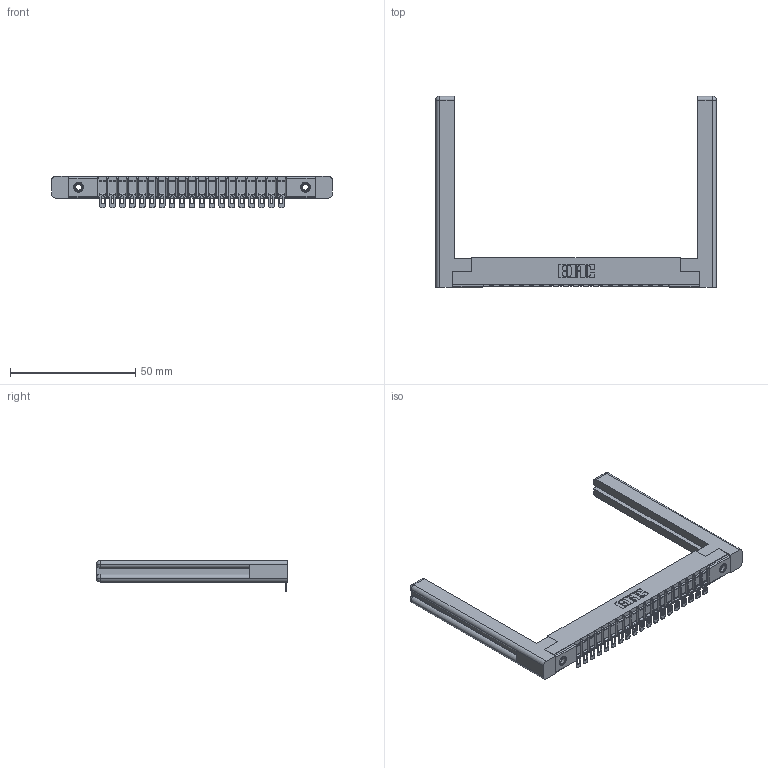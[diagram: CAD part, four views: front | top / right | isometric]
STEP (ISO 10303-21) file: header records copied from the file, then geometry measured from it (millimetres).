
FILE_DESCRIPTION (( 'STEP AP203' ), '1' );
FILE_NAME ('307-019-554-158.STEP', '2019-09-04T22:49:40', ( '' ), ( '' ), 'SwSTEP 2.0', 'SolidWorks 2016', '' );
FILE_SCHEMA (( 'CONFIG_CONTROL_DESIGN' ));
Length unit declared in the file: inch
Products named in the file (5): 307-290-002_554; 345-250-001_345-250-001-102; 307-019-554-158; 307-220-058; 307 Part_.156 Dia Mounting Holes
Assembly tree (24 placements, depth 2):
  307-019-554-158
    307 Part_.156 Dia Mounting Holes
    307-290-002_554  x19
    307-220-058  x2
    345-250-001_345-250-001-102  x2
Bounding box: 111.91 x 76.33 x 12.52 mm (x, y, z)
Volume: 15071.9 mm3; surface area: 18383.3 mm2
Topology: 24 solids, 24 shells, 1819 faces, 5484 edges, 3588 vertices
Faces by surface type: plane 1028, cylinder 727, sphere 40, torus 12, cone 12
Entity records: 22722 total; most frequent: CARTESIAN_POINT 3837, ORIENTED_EDGE 3766, DIRECTION 3705, EDGE_CURVE 1883, LINE 1421, VECTOR 1421, VERTEX_POINT 1220, AXIS2_PLACEMENT_3D 1142
